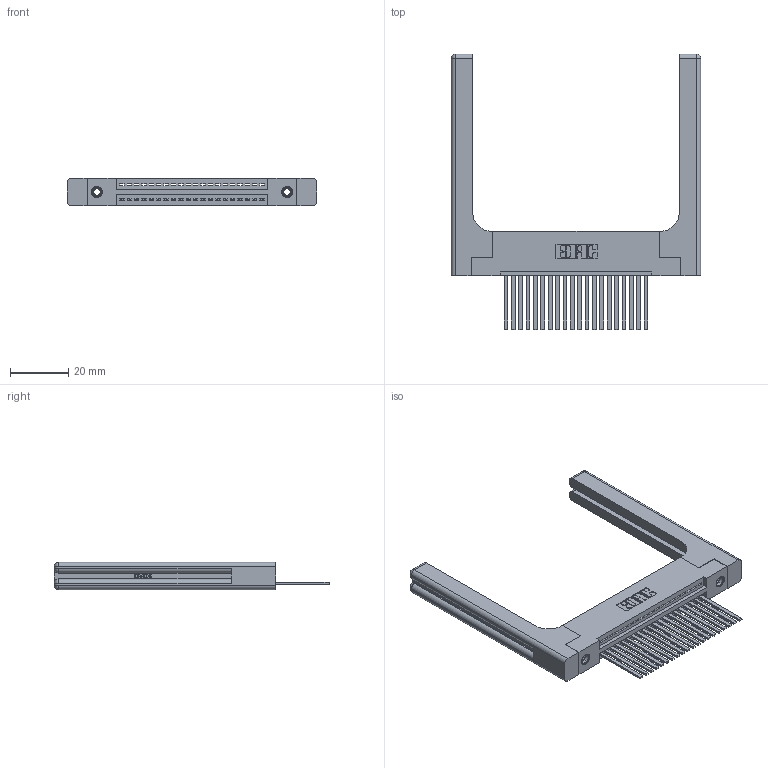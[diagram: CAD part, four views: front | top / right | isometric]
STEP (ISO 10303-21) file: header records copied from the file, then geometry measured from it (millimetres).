
FILE_DESCRIPTION (( 'STEP AP203' ), '1' );
FILE_NAME ('345-020-544-158.STEP', '2019-10-04T21:12:36', ( '' ), ( '' ), 'SwSTEP 2.0', 'SolidWorks 2016', '' );
FILE_SCHEMA (( 'CONFIG_CONTROL_DESIGN' ));
Length unit declared in the file: inch
Products named in the file (5): 345-220-058_345-220-058; 345-250-001_345-250-001-102; 345-020-544-158; 345 Part_Flush Mounting Lugs - 0.156 Dia-TH; 345-292-001_345-293-144
Assembly tree (25 placements, depth 2):
  345-020-544-158
    345 Part_Flush Mounting Lugs - 0.156 Dia-TH
    345-292-001_345-293-144  x20
    345-250-001_345-250-001-102  x2
    345-220-058_345-220-058  x2
Bounding box: 85.83 x 94.92 x 9.4 mm (x, y, z)
Volume: 16708.3 mm3; surface area: 16603.4 mm2
Topology: 25 solids, 25 shells, 1422 faces, 4167 edges, 2730 vertices
Faces by surface type: plane 948, cylinder 414, bspline 36, cone 12, sphere 8, torus 4
Entity records: 23012 total; most frequent: CARTESIAN_POINT 4957, ORIENTED_EDGE 3708, DIRECTION 3306, EDGE_CURVE 1854, LINE 1554, VECTOR 1554, VERTEX_POINT 1226, AXIS2_PLACEMENT_3D 876
